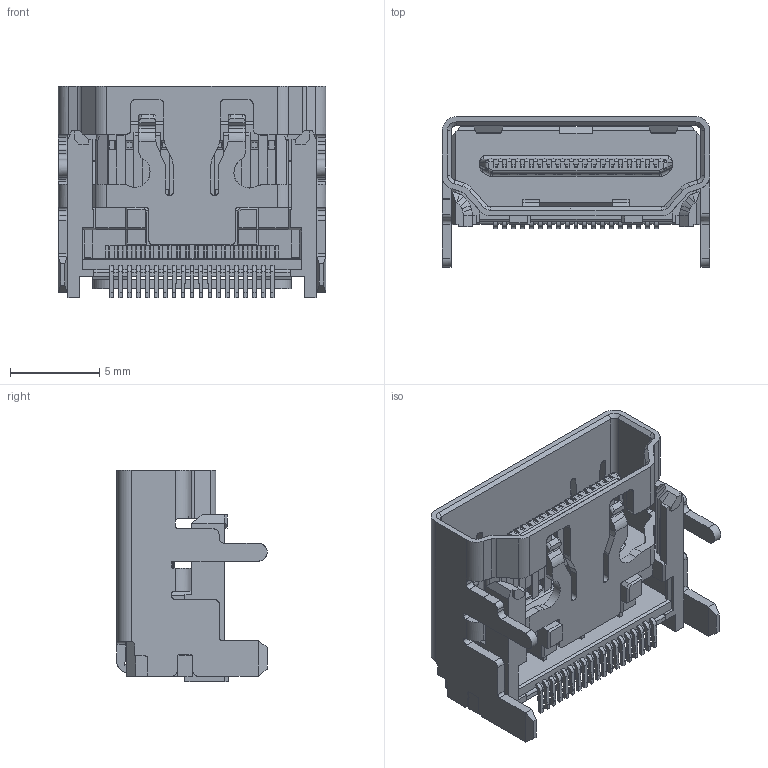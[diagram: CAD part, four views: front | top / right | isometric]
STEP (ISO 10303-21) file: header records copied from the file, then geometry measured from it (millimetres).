
FILE_DESCRIPTION (( 'STEP AP214' ), '1' );
FILE_NAME ('694D119-165-011.STEP', '2021-01-13T16:12:02', ( '' ), ( '' ), 'SwSTEP 2.0', 'SolidWorks 2020', '' );
FILE_SCHEMA (( 'AUTOMOTIVE_DESIGN' ));
Length unit declared in the file: millimetre
Products named in the file (3): 694D119-165-011; Insulator 694D119-X65-011; Shell 694D119-X65-011
Assembly tree (2 placements, depth 2):
  694D119-165-011
    Insulator 694D119-X65-011
    Shell 694D119-X65-011
Bounding box: 15 x 8.43 x 11.87 mm (x, y, z)
Volume: 450.5 mm3; surface area: 1558.4 mm2
Topology: 2 solids, 2 shells, 1694 faces, 4780 edges, 3097 vertices
Faces by surface type: plane 1301, cylinder 359, cone 14, bspline 9, torus 7, sphere 4
Entity records: 60404 total; most frequent: CARTESIAN_POINT 14171, ORIENTED_EDGE 9556, DIRECTION 6796, EDGE_CURVE 4778, VERTEX_POINT 3097, VECTOR 2606, LINE 2606, AXIS2_PLACEMENT_3D 2095
